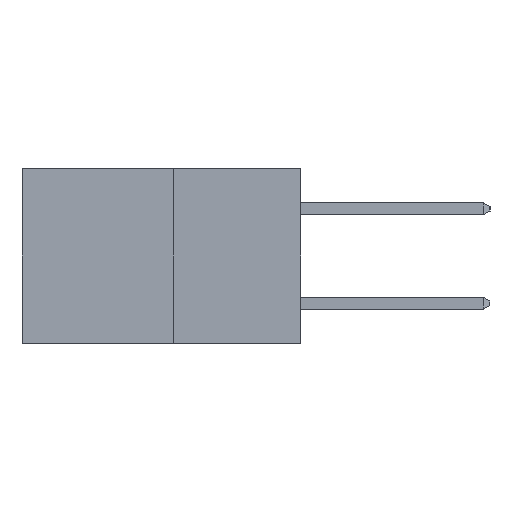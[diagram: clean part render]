
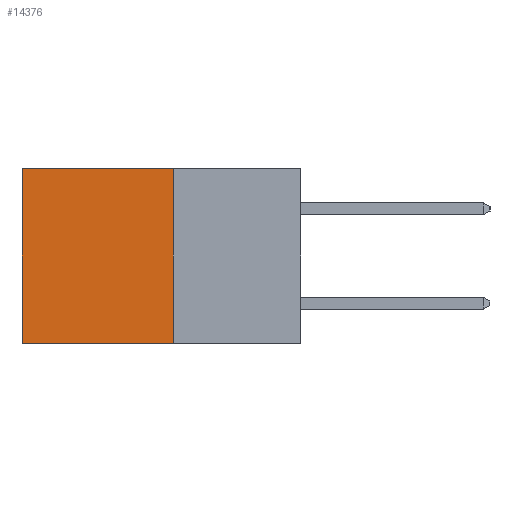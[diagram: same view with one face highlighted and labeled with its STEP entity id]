
A CAD part, left-side view. The second image highlights one B-rep face of the part: STEP entity #14376.
In plain terms, the highlighted planar face has unit normal (-1, 0, 0).
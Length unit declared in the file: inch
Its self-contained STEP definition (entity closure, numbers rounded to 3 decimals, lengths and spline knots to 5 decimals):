
#965 = CARTESIAN_POINT ( 'NONE',  ( 0.277, 0.59, -0.37 ) ) ;
#1226 = VECTOR ( 'NONE', #9535, 39.37008 ) ;
#1245 = ORIENTED_EDGE ( 'NONE', *, *, #11354, .F. ) ;
#1391 = CARTESIAN_POINT ( 'NONE',  ( 0.277, 0.27, -0.37 ) ) ;
#1863 = LINE ( 'NONE', #11175, #4888 ) ;
#2232 = VERTEX_POINT ( 'NONE', #8957 ) ;
#2477 = CARTESIAN_POINT ( 'NONE',  ( 0.277, 0.27, 0. ) ) ;
#4779 = DIRECTION ( 'NONE',  ( 1., 0., 0. ) ) ;
#4804 = DIRECTION ( 'NONE',  ( 0., 1., 0. ) ) ;
#4888 = VECTOR ( 'NONE', #4804, 39.37008 ) ;
#7396 = LINE ( 'NONE', #965, #7815 ) ;
#7716 = EDGE_CURVE ( 'NONE', #9198, #15508, #8501, .T. ) ;
#7815 = VECTOR ( 'NONE', #10026, 39.37008 ) ;
#8103 = ORIENTED_EDGE ( 'NONE', *, *, #7716, .T. ) ;
#8333 = CARTESIAN_POINT ( 'NONE',  ( 0.277, 0.27, -0.37 ) ) ;
#8501 = LINE ( 'NONE', #9468, #1226 ) ;
#8546 = CARTESIAN_POINT ( 'NONE',  ( 0.277, 0.59, 0. ) ) ;
#8957 = CARTESIAN_POINT ( 'NONE',  ( 0.277, 0.59, -0.37 ) ) ;
#9095 = FACE_OUTER_BOUND ( 'NONE', #12420, .T. ) ;
#9198 = VERTEX_POINT ( 'NONE', #2477 ) ;
#9468 = CARTESIAN_POINT ( 'NONE',  ( 0.277, 0.27, 0. ) ) ;
#9535 = DIRECTION ( 'NONE',  ( 0., 1., 0. ) ) ;
#9886 = CARTESIAN_POINT ( 'NONE',  ( 0.277, 0.27, -0.37 ) ) ;
#10026 = DIRECTION ( 'NONE',  ( 0., 0., -1. ) ) ;
#11175 = CARTESIAN_POINT ( 'NONE',  ( 0.277, 0.27, -0.37 ) ) ;
#11354 = EDGE_CURVE ( 'NONE', #9198, #14780, #14714, .T. ) ;
#11550 = VECTOR ( 'NONE', #13387, 39.37008 ) ;
#12405 = PLANE ( 'NONE',  #14296 ) ;
#12420 = EDGE_LOOP ( 'NONE', ( #13610, #13994, #1245, #8103 ) ) ;
#13387 = DIRECTION ( 'NONE',  ( 0., 0., -1. ) ) ;
#13603 = DIRECTION ( 'NONE',  ( 0., 0., -1. ) ) ;
#13610 = ORIENTED_EDGE ( 'NONE', *, *, #15652, .T. ) ;
#13991 = EDGE_CURVE ( 'NONE', #14780, #2232, #1863, .T. ) ;
#13994 = ORIENTED_EDGE ( 'NONE', *, *, #13991, .F. ) ;
#14296 = AXIS2_PLACEMENT_3D ( 'NONE', #9886, #4779, #13603 ) ;
#14376 = ADVANCED_FACE ( 'NONE', ( #9095 ), #12405, .F. ) ;
#14714 = LINE ( 'NONE', #8333, #11550 ) ;
#14780 = VERTEX_POINT ( 'NONE', #1391 ) ;
#15508 = VERTEX_POINT ( 'NONE', #8546 ) ;
#15652 = EDGE_CURVE ( 'NONE', #15508, #2232, #7396, .T. ) ;
